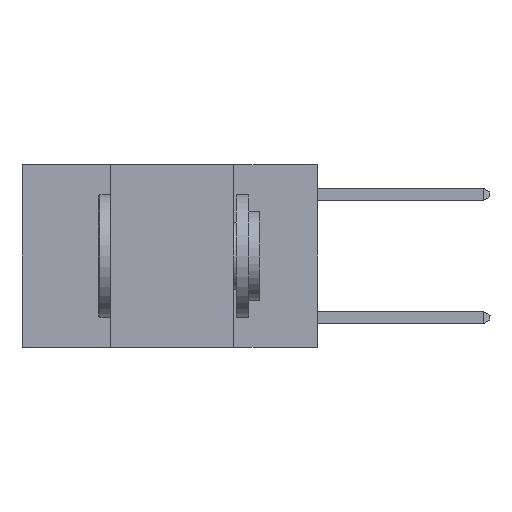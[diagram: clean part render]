
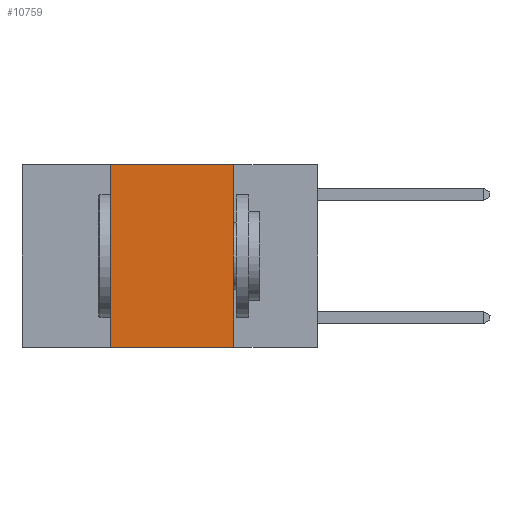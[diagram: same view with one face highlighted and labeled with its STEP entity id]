
A CAD part, left-side view. The second image highlights one B-rep face of the part: STEP entity #10759.
In plain terms, the highlighted planar face has unit normal (-1, 0, 0).
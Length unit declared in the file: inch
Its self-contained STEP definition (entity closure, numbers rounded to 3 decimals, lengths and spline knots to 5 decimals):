
#745 = EDGE_CURVE ( 'NONE', #23141, #23488, #4359, .T. ) ;
#3540 = EDGE_CURVE ( 'NONE', #23141, #15508, #11638, .T. ) ;
#3800 = EDGE_LOOP ( 'NONE', ( #19982, #6549, #11946, #8143 ) ) ;
#3943 = CARTESIAN_POINT ( 'NONE',  ( 0., 0.6, -0.37 ) ) ;
#4359 = LINE ( 'NONE', #3943, #4998 ) ;
#4754 = CARTESIAN_POINT ( 'NONE',  ( 0., 0.17, -0.37 ) ) ;
#4972 = DIRECTION ( 'NONE',  ( 0., -1., 0. ) ) ;
#4998 = VECTOR ( 'NONE', #23730, 39.37008 ) ;
#5646 = DIRECTION ( 'NONE',  ( 0., 0., -1. ) ) ;
#6127 = VECTOR ( 'NONE', #15432, 39.37008 ) ;
#6549 = ORIENTED_EDGE ( 'NONE', *, *, #22221, .F. ) ;
#6784 = CARTESIAN_POINT ( 'NONE',  ( 0., 0.42, 0. ) ) ;
#8143 = ORIENTED_EDGE ( 'NONE', *, *, #745, .T. ) ;
#9004 = CARTESIAN_POINT ( 'NONE',  ( 0., 0.6, 0. ) ) ;
#9253 = CARTESIAN_POINT ( 'NONE',  ( 0., 0.17, 0. ) ) ;
#10515 = LINE ( 'NONE', #15531, #20674 ) ;
#10759 = ADVANCED_FACE ( 'NONE', ( #23737 ), #15877, .F. ) ;
#11638 = LINE ( 'NONE', #23372, #6127 ) ;
#11946 = ORIENTED_EDGE ( 'NONE', *, *, #3540, .F. ) ;
#13235 = EDGE_CURVE ( 'NONE', #24383, #23488, #10515, .T. ) ;
#15432 = DIRECTION ( 'NONE',  ( 0., 0., 1. ) ) ;
#15508 = VERTEX_POINT ( 'NONE', #6784 ) ;
#15531 = CARTESIAN_POINT ( 'NONE',  ( 0., 0.17, 0. ) ) ;
#15877 = PLANE ( 'NONE',  #24908 ) ;
#15970 = VECTOR ( 'NONE', #4972, 39.37008 ) ;
#17894 = DIRECTION ( 'NONE',  ( 1., 0., 0. ) ) ;
#18087 = CARTESIAN_POINT ( 'NONE',  ( 0., 0.42, -0.37 ) ) ;
#19982 = ORIENTED_EDGE ( 'NONE', *, *, #13235, .F. ) ;
#20674 = VECTOR ( 'NONE', #23470, 39.37008 ) ;
#21305 = LINE ( 'NONE', #9004, #15970 ) ;
#22221 = EDGE_CURVE ( 'NONE', #15508, #24383, #21305, .T. ) ;
#23141 = VERTEX_POINT ( 'NONE', #18087 ) ;
#23372 = CARTESIAN_POINT ( 'NONE',  ( 0., 0.42, 0. ) ) ;
#23470 = DIRECTION ( 'NONE',  ( 0., 0., -1. ) ) ;
#23488 = VERTEX_POINT ( 'NONE', #4754 ) ;
#23730 = DIRECTION ( 'NONE',  ( 0., -1., 0. ) ) ;
#23737 = FACE_OUTER_BOUND ( 'NONE', #3800, .T. ) ;
#23797 = CARTESIAN_POINT ( 'NONE',  ( 0., 0.6, 0. ) ) ;
#24383 = VERTEX_POINT ( 'NONE', #9253 ) ;
#24908 = AXIS2_PLACEMENT_3D ( 'NONE', #23797, #17894, #5646 ) ;
